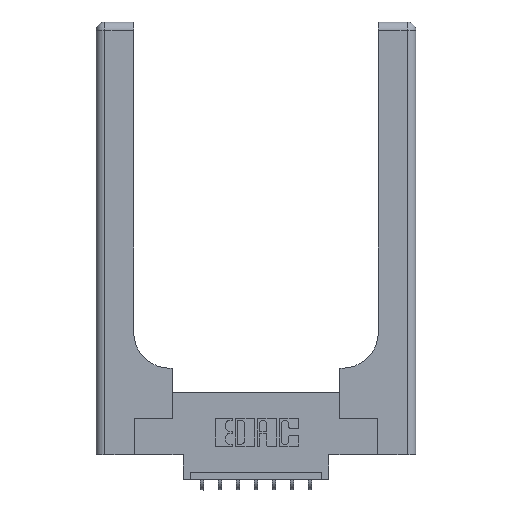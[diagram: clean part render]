
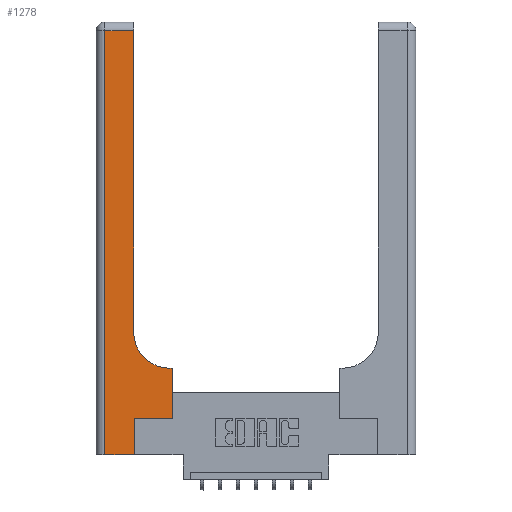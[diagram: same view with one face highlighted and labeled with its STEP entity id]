
A CAD part, top view. The second image highlights one B-rep face of the part: STEP entity #1278.
In plain terms, the highlighted planar face has unit normal (0, 0, 1).
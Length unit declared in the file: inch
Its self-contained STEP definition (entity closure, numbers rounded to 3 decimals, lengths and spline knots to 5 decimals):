
#269 = CARTESIAN_POINT ( 'NONE',  ( 0., 2.94, 0.37 ) ) ;
#745 = LINE ( 'NONE', #5297, #897 ) ;
#897 = VECTOR ( 'NONE', #6505, 39.37008 ) ;
#904 = ORIENTED_EDGE ( 'NONE', *, *, #5445, .T. ) ;
#1278 = ADVANCED_FACE ( 'NONE', ( #3254 ), #4516, .F. ) ;
#1359 = EDGE_CURVE ( 'NONE', #13672, #5765, #6714, .T. ) ;
#1619 = CARTESIAN_POINT ( 'NONE',  ( 0.51, 0.85, 0.37 ) ) ;
#1743 = CIRCLE ( 'NONE', #2453, 0.25 ) ;
#1910 = DIRECTION ( 'NONE',  ( 1., 0., 0. ) ) ;
#1997 = LINE ( 'NONE', #9930, #10271 ) ;
#2157 = VECTOR ( 'NONE', #3331, 39.37008 ) ;
#2453 = AXIS2_PLACEMENT_3D ( 'NONE', #1619, #7406, #1910 ) ;
#2636 = AXIS2_PLACEMENT_3D ( 'NONE', #13825, #12702, #5810 ) ;
#3007 = VECTOR ( 'NONE', #9618, 39.37008 ) ;
#3192 = CARTESIAN_POINT ( 'NONE',  ( 0.26, 3., 0.37 ) ) ;
#3254 = FACE_OUTER_BOUND ( 'NONE', #14466, .T. ) ;
#3331 = DIRECTION ( 'NONE',  ( 0., -1., 0. ) ) ;
#3430 = DIRECTION ( 'NONE',  ( 1., 0., 0. ) ) ;
#3655 = ORIENTED_EDGE ( 'NONE', *, *, #6844, .T. ) ;
#4105 = CARTESIAN_POINT ( 'NONE',  ( 0.06, 2.94, 0.37 ) ) ;
#4443 = CARTESIAN_POINT ( 'NONE',  ( 0.06, 3., 0.37 ) ) ;
#4516 = PLANE ( 'NONE',  #2636 ) ;
#4705 = LINE ( 'NONE', #6898, #12444 ) ;
#4785 = CARTESIAN_POINT ( 'NONE',  ( 0.528, 0.6, 0.37 ) ) ;
#5297 = CARTESIAN_POINT ( 'NONE',  ( 0.26, 0.6, 0.37 ) ) ;
#5445 = EDGE_CURVE ( 'NONE', #8456, #13865, #12122, .T. ) ;
#5760 = CARTESIAN_POINT ( 'NONE',  ( 0.528, 0.25, 0.37 ) ) ;
#5765 = VERTEX_POINT ( 'NONE', #6549 ) ;
#5810 = DIRECTION ( 'NONE',  ( -1., 0., 0. ) ) ;
#6138 = VECTOR ( 'NONE', #12979, 39.37008 ) ;
#6505 = DIRECTION ( 'NONE',  ( -1., 0., 0. ) ) ;
#6549 = CARTESIAN_POINT ( 'NONE',  ( 0.06, 0., 0.37 ) ) ;
#6614 = VERTEX_POINT ( 'NONE', #10373 ) ;
#6714 = LINE ( 'NONE', #4443, #2157 ) ;
#6844 = EDGE_CURVE ( 'NONE', #8014, #8456, #1743, .T. ) ;
#6898 = CARTESIAN_POINT ( 'NONE',  ( 0.265, 0.25, 0.37 ) ) ;
#7226 = CARTESIAN_POINT ( 'NONE',  ( 0.528, 0.25, 0.37 ) ) ;
#7249 = LINE ( 'NONE', #269, #3007 ) ;
#7406 = DIRECTION ( 'NONE',  ( 0., 0., -1. ) ) ;
#7431 = ORIENTED_EDGE ( 'NONE', *, *, #14085, .T. ) ;
#8014 = VERTEX_POINT ( 'NONE', #14725 ) ;
#8173 = ORIENTED_EDGE ( 'NONE', *, *, #14333, .T. ) ;
#8456 = VERTEX_POINT ( 'NONE', #9416 ) ;
#8628 = LINE ( 'NONE', #11072, #12167 ) ;
#9416 = CARTESIAN_POINT ( 'NONE',  ( 0.26, 0.85, 0.37 ) ) ;
#9516 = LINE ( 'NONE', #7226, #6138 ) ;
#9618 = DIRECTION ( 'NONE',  ( -1., 0., 0. ) ) ;
#9930 = CARTESIAN_POINT ( 'NONE',  ( 0.265, 0., 0.37 ) ) ;
#10182 = EDGE_CURVE ( 'NONE', #5765, #6614, #8628, .T. ) ;
#10254 = VERTEX_POINT ( 'NONE', #10289 ) ;
#10271 = VECTOR ( 'NONE', #14808, 39.37008 ) ;
#10289 = CARTESIAN_POINT ( 'NONE',  ( 0.265, 0.25, 0.37 ) ) ;
#10373 = CARTESIAN_POINT ( 'NONE',  ( 0.265, 0., 0.37 ) ) ;
#10381 = EDGE_CURVE ( 'NONE', #13865, #13672, #7249, .T. ) ;
#10913 = VECTOR ( 'NONE', #13463, 39.37008 ) ;
#11072 = CARTESIAN_POINT ( 'NONE',  ( 0., 0., 0.37 ) ) ;
#11139 = DIRECTION ( 'NONE',  ( 1., 0., 0. ) ) ;
#11195 = ORIENTED_EDGE ( 'NONE', *, *, #10381, .T. ) ;
#12122 = LINE ( 'NONE', #3192, #10913 ) ;
#12167 = VECTOR ( 'NONE', #11139, 39.37008 ) ;
#12323 = ORIENTED_EDGE ( 'NONE', *, *, #14373, .T. ) ;
#12436 = VERTEX_POINT ( 'NONE', #4785 ) ;
#12444 = VECTOR ( 'NONE', #3430, 39.37008 ) ;
#12702 = DIRECTION ( 'NONE',  ( 0., 0., -1. ) ) ;
#12768 = VERTEX_POINT ( 'NONE', #5760 ) ;
#12979 = DIRECTION ( 'NONE',  ( 0., 1., 0. ) ) ;
#13077 = ORIENTED_EDGE ( 'NONE', *, *, #10182, .T. ) ;
#13245 = EDGE_CURVE ( 'NONE', #12768, #12436, #9516, .T. ) ;
#13463 = DIRECTION ( 'NONE',  ( 0., 1., 0. ) ) ;
#13672 = VERTEX_POINT ( 'NONE', #4105 ) ;
#13825 = CARTESIAN_POINT ( 'NONE',  ( 0., 3., 0.37 ) ) ;
#13865 = VERTEX_POINT ( 'NONE', #14831 ) ;
#13996 = ORIENTED_EDGE ( 'NONE', *, *, #1359, .T. ) ;
#14085 = EDGE_CURVE ( 'NONE', #10254, #12768, #4705, .T. ) ;
#14333 = EDGE_CURVE ( 'NONE', #12436, #8014, #745, .T. ) ;
#14355 = ORIENTED_EDGE ( 'NONE', *, *, #13245, .T. ) ;
#14373 = EDGE_CURVE ( 'NONE', #6614, #10254, #1997, .T. ) ;
#14466 = EDGE_LOOP ( 'NONE', ( #904, #11195, #13996, #13077, #12323, #7431, #14355, #8173, #3655 ) ) ;
#14725 = CARTESIAN_POINT ( 'NONE',  ( 0.51, 0.6, 0.37 ) ) ;
#14808 = DIRECTION ( 'NONE',  ( 0., 1., 0. ) ) ;
#14831 = CARTESIAN_POINT ( 'NONE',  ( 0.26, 2.94, 0.37 ) ) ;
